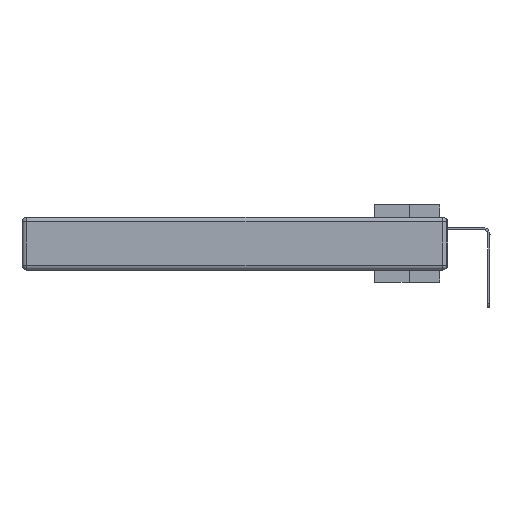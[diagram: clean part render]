
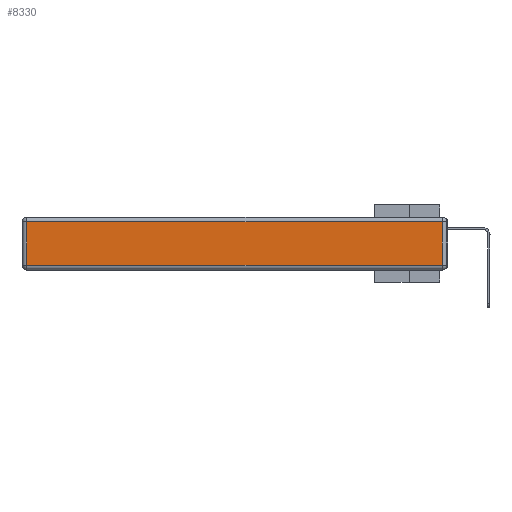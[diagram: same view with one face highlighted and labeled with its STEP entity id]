
A CAD part, left-side view. The second image highlights one B-rep face of the part: STEP entity #8330.
In plain terms, the highlighted planar face has unit normal (-1, 0, 0).
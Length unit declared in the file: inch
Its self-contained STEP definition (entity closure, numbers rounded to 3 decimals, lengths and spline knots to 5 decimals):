
#1086 = CARTESIAN_POINT ( 'NONE',  ( 0., 2.72, -0.03 ) ) ;
#2146 = FACE_OUTER_BOUND ( 'NONE', #21835, .T. ) ;
#2684 = DIRECTION ( 'NONE',  ( 0., 0., 1. ) ) ;
#2923 = DIRECTION ( 'NONE',  ( 0., 1., 0. ) ) ;
#3037 = DIRECTION ( 'NONE',  ( 0., -1., 0. ) ) ;
#3141 = VERTEX_POINT ( 'NONE', #15279 ) ;
#4423 = VERTEX_POINT ( 'NONE', #1086 ) ;
#5273 = VERTEX_POINT ( 'NONE', #7715 ) ;
#5648 = LINE ( 'NONE', #28402, #26896 ) ;
#5701 = DIRECTION ( 'NONE',  ( -1., 0., 0. ) ) ;
#7715 = CARTESIAN_POINT ( 'NONE',  ( 0., 2.72, -0.313 ) ) ;
#7876 = VECTOR ( 'NONE', #2923, 39.37008 ) ;
#8330 = ADVANCED_FACE ( 'NONE', ( #2146 ), #19921, .T. ) ;
#9958 = VECTOR ( 'NONE', #3037, 39.37008 ) ;
#11269 = ORIENTED_EDGE ( 'NONE', *, *, #28936, .T. ) ;
#11560 = EDGE_CURVE ( 'NONE', #5273, #37113, #17221, .T. ) ;
#12037 = CARTESIAN_POINT ( 'NONE',  ( 0., 2.72, -0.343 ) ) ;
#12402 = ORIENTED_EDGE ( 'NONE', *, *, #33886, .T. ) ;
#12483 = ORIENTED_EDGE ( 'NONE', *, *, #13387, .T. ) ;
#13387 = EDGE_CURVE ( 'NONE', #37113, #3141, #5648, .T. ) ;
#14915 = ORIENTED_EDGE ( 'NONE', *, *, #11560, .T. ) ;
#15279 = CARTESIAN_POINT ( 'NONE',  ( 0., 0.03, -0.03 ) ) ;
#16037 = CARTESIAN_POINT ( 'NONE',  ( 0., 0.03, -0.313 ) ) ;
#17221 = LINE ( 'NONE', #34681, #9958 ) ;
#19631 = DIRECTION ( 'NONE',  ( 0., 0., 1. ) ) ;
#19921 = PLANE ( 'NONE',  #25950 ) ;
#20604 = LINE ( 'NONE', #31421, #7876 ) ;
#21835 = EDGE_LOOP ( 'NONE', ( #14915, #12483, #12402, #11269 ) ) ;
#25950 = AXIS2_PLACEMENT_3D ( 'NONE', #37233, #5701, #2684 ) ;
#26896 = VECTOR ( 'NONE', #19631, 39.37008 ) ;
#28402 = CARTESIAN_POINT ( 'NONE',  ( 0., 0.03, -0.343 ) ) ;
#28936 = EDGE_CURVE ( 'NONE', #4423, #5273, #32642, .T. ) ;
#31421 = CARTESIAN_POINT ( 'NONE',  ( 0., 2.75, -0.03 ) ) ;
#32642 = LINE ( 'NONE', #12037, #37154 ) ;
#33886 = EDGE_CURVE ( 'NONE', #3141, #4423, #20604, .T. ) ;
#34681 = CARTESIAN_POINT ( 'NONE',  ( 0., 0., -0.313 ) ) ;
#35916 = DIRECTION ( 'NONE',  ( 0., 0., -1. ) ) ;
#37113 = VERTEX_POINT ( 'NONE', #16037 ) ;
#37154 = VECTOR ( 'NONE', #35916, 39.37008 ) ;
#37233 = CARTESIAN_POINT ( 'NONE',  ( 0., 0., -0.343 ) ) ;
